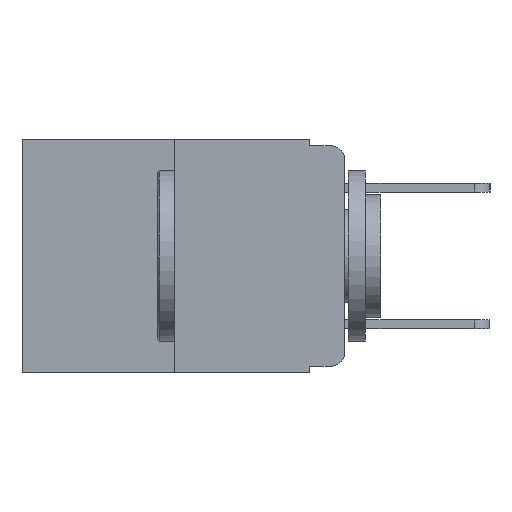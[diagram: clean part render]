
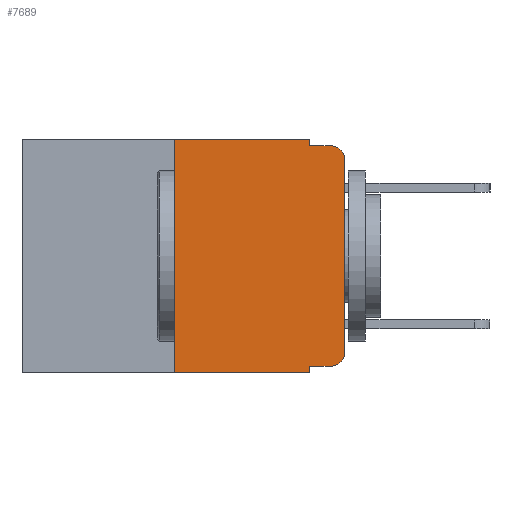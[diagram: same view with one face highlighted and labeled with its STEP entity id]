
A CAD part, left-side view. The second image highlights one B-rep face of the part: STEP entity #7689.
In plain terms, the highlighted planar face has unit normal (-1, 0, 0).
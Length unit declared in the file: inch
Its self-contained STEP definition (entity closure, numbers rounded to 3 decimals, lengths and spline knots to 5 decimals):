
#32 = CARTESIAN_POINT ( 'NONE',  ( 0., 0.051, 0. ) ) ;
#112 = CIRCLE ( 'NONE', #14133, 0.02 ) ;
#228 = LINE ( 'NONE', #32, #11979 ) ;
#913 = VECTOR ( 'NONE', #4139, 39.37008 ) ;
#923 = VERTEX_POINT ( 'NONE', #8647 ) ;
#936 = ORIENTED_EDGE ( 'NONE', *, *, #11792, .F. ) ;
#1108 = DIRECTION ( 'NONE',  ( 0., 0., -1. ) ) ;
#1248 = CARTESIAN_POINT ( 'NONE',  ( 0., 0.02, -0.03 ) ) ;
#1692 = VERTEX_POINT ( 'NONE', #4587 ) ;
#2094 = DIRECTION ( 'NONE',  ( 0., -1., 0. ) ) ;
#2232 = CARTESIAN_POINT ( 'NONE',  ( 0., 0., -0.03 ) ) ;
#2318 = CARTESIAN_POINT ( 'NONE',  ( 0., 0.02, -0.313 ) ) ;
#2529 = DIRECTION ( 'NONE',  ( 0., 0., -1. ) ) ;
#2542 = LINE ( 'NONE', #11298, #8085 ) ;
#2776 = VERTEX_POINT ( 'NONE', #5803 ) ;
#2976 = VERTEX_POINT ( 'NONE', #9753 ) ;
#3293 = CARTESIAN_POINT ( 'NONE',  ( 0., 0.051, -0.333 ) ) ;
#3555 = DIRECTION ( 'NONE',  ( 0., 0., -1. ) ) ;
#3760 = CARTESIAN_POINT ( 'NONE',  ( 0., 0.02, -0.01 ) ) ;
#3889 = ORIENTED_EDGE ( 'NONE', *, *, #6026, .T. ) ;
#3990 = DIRECTION ( 'NONE',  ( 0., 0., -1. ) ) ;
#4072 = FACE_OUTER_BOUND ( 'NONE', #4686, .T. ) ;
#4139 = DIRECTION ( 'NONE',  ( 0., 0., 1. ) ) ;
#4497 = ORIENTED_EDGE ( 'NONE', *, *, #5230, .T. ) ;
#4522 = CARTESIAN_POINT ( 'NONE',  ( 0., 0.02, -0.333 ) ) ;
#4587 = CARTESIAN_POINT ( 'NONE',  ( 0., 0.051, -0.343 ) ) ;
#4591 = LINE ( 'NONE', #3293, #10082 ) ;
#4680 = LINE ( 'NONE', #11392, #10151 ) ;
#4686 = EDGE_LOOP ( 'NONE', ( #3889, #4497, #4713, #6144, #11486, #13515, #8581, #936, #9723, #12832 ) ) ;
#4713 = ORIENTED_EDGE ( 'NONE', *, *, #14238, .F. ) ;
#5064 = VECTOR ( 'NONE', #6208, 39.37008 ) ;
#5230 = EDGE_CURVE ( 'NONE', #9731, #10105, #10468, .T. ) ;
#5326 = DIRECTION ( 'NONE',  ( 1., 0., 0. ) ) ;
#5803 = CARTESIAN_POINT ( 'NONE',  ( 0., 0.051, 0. ) ) ;
#5933 = EDGE_CURVE ( 'NONE', #13822, #1692, #2542, .T. ) ;
#5984 = LINE ( 'NONE', #12534, #11494 ) ;
#6026 = EDGE_CURVE ( 'NONE', #2976, #9731, #4680, .T. ) ;
#6144 = ORIENTED_EDGE ( 'NONE', *, *, #13637, .F. ) ;
#6208 = DIRECTION ( 'NONE',  ( 0., -1., 0. ) ) ;
#6488 = DIRECTION ( 'NONE',  ( 0., -1., 0. ) ) ;
#7689 = ADVANCED_FACE ( 'NONE', ( #4072 ), #9641, .F. ) ;
#8085 = VECTOR ( 'NONE', #11265, 39.37008 ) ;
#8264 = CARTESIAN_POINT ( 'NONE',  ( 0., 0.051, 0. ) ) ;
#8392 = DIRECTION ( 'NONE',  ( 0., 0., 1. ) ) ;
#8401 = CARTESIAN_POINT ( 'NONE',  ( 0., 0.25, -0.343 ) ) ;
#8581 = ORIENTED_EDGE ( 'NONE', *, *, #5933, .T. ) ;
#8647 = CARTESIAN_POINT ( 'NONE',  ( 0., 0.051, -0.01 ) ) ;
#8709 = LINE ( 'NONE', #8264, #11347 ) ;
#9185 = CARTESIAN_POINT ( 'NONE',  ( 0., 0.25, 0. ) ) ;
#9418 = DIRECTION ( 'NONE',  ( -1., 0., 0. ) ) ;
#9641 = PLANE ( 'NONE',  #13211 ) ;
#9723 = ORIENTED_EDGE ( 'NONE', *, *, #11153, .T. ) ;
#9731 = VERTEX_POINT ( 'NONE', #2232 ) ;
#9753 = CARTESIAN_POINT ( 'NONE',  ( 0., 0., -0.313 ) ) ;
#9836 = VERTEX_POINT ( 'NONE', #9185 ) ;
#9861 = EDGE_CURVE ( 'NONE', #11091, #2976, #112, .T. ) ;
#10082 = VECTOR ( 'NONE', #2094, 39.37008 ) ;
#10105 = VERTEX_POINT ( 'NONE', #3760 ) ;
#10151 = VECTOR ( 'NONE', #8392, 39.37008 ) ;
#10230 = DIRECTION ( 'NONE',  ( -1., 0., 0. ) ) ;
#10468 = CIRCLE ( 'NONE', #12814, 0.02 ) ;
#10597 = CARTESIAN_POINT ( 'NONE',  ( 0., 0.473, 0. ) ) ;
#10711 = CARTESIAN_POINT ( 'NONE',  ( 0., 0.25, 0. ) ) ;
#10762 = LINE ( 'NONE', #12294, #5064 ) ;
#11091 = VERTEX_POINT ( 'NONE', #4522 ) ;
#11153 = EDGE_CURVE ( 'NONE', #13520, #11091, #4591, .T. ) ;
#11265 = DIRECTION ( 'NONE',  ( 0., -1., 0. ) ) ;
#11298 = CARTESIAN_POINT ( 'NONE',  ( 0., 0.473, -0.343 ) ) ;
#11347 = VECTOR ( 'NONE', #1108, 39.37008 ) ;
#11392 = CARTESIAN_POINT ( 'NONE',  ( 0., 0., 0. ) ) ;
#11486 = ORIENTED_EDGE ( 'NONE', *, *, #13807, .F. ) ;
#11494 = VECTOR ( 'NONE', #6488, 39.37008 ) ;
#11792 = EDGE_CURVE ( 'NONE', #13520, #1692, #228, .T. ) ;
#11979 = VECTOR ( 'NONE', #3990, 39.37008 ) ;
#11996 = CARTESIAN_POINT ( 'NONE',  ( 0., 0.051, -0.333 ) ) ;
#12091 = LINE ( 'NONE', #10711, #913 ) ;
#12294 = CARTESIAN_POINT ( 'NONE',  ( 0., 0.473, 0. ) ) ;
#12527 = DIRECTION ( 'NONE',  ( 0., 0., -1. ) ) ;
#12534 = CARTESIAN_POINT ( 'NONE',  ( 0., 0.051, -0.01 ) ) ;
#12814 = AXIS2_PLACEMENT_3D ( 'NONE', #1248, #9418, #2529 ) ;
#12832 = ORIENTED_EDGE ( 'NONE', *, *, #9861, .T. ) ;
#13012 = EDGE_CURVE ( 'NONE', #13822, #9836, #12091, .T. ) ;
#13211 = AXIS2_PLACEMENT_3D ( 'NONE', #10597, #5326, #12527 ) ;
#13515 = ORIENTED_EDGE ( 'NONE', *, *, #13012, .F. ) ;
#13520 = VERTEX_POINT ( 'NONE', #11996 ) ;
#13637 = EDGE_CURVE ( 'NONE', #2776, #923, #8709, .T. ) ;
#13807 = EDGE_CURVE ( 'NONE', #9836, #2776, #10762, .T. ) ;
#13822 = VERTEX_POINT ( 'NONE', #8401 ) ;
#14133 = AXIS2_PLACEMENT_3D ( 'NONE', #2318, #10230, #3555 ) ;
#14238 = EDGE_CURVE ( 'NONE', #923, #10105, #5984, .T. ) ;
